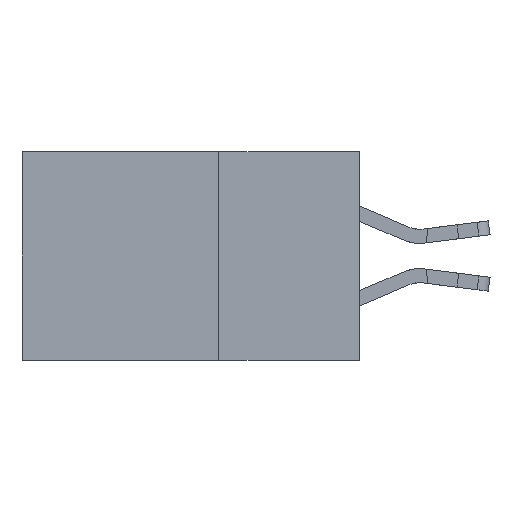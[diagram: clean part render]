
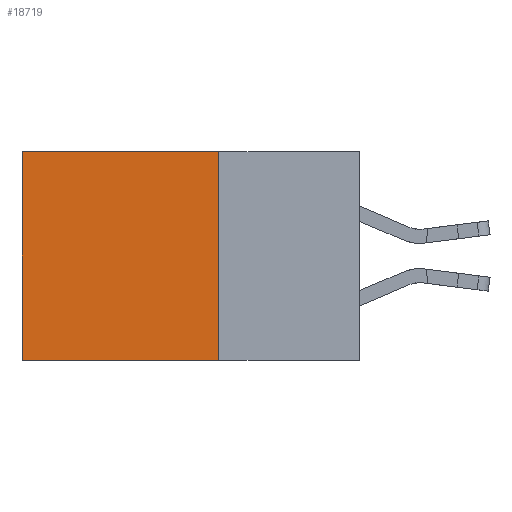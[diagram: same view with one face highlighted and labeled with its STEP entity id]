
A CAD part, left-side view. The second image highlights one B-rep face of the part: STEP entity #18719.
In plain terms, the highlighted planar face has unit normal (-1, 0, 0).
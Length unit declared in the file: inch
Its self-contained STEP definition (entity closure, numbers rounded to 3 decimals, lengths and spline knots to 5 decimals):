
#440 = CARTESIAN_POINT ( 'NONE',  ( 0.2875, 0.25, -0.37 ) ) ;
#581 = DIRECTION ( 'NONE',  ( 0., 1., 0. ) ) ;
#1098 = ORIENTED_EDGE ( 'NONE', *, *, #12425, .T. ) ;
#3612 = CARTESIAN_POINT ( 'NONE',  ( 0.2875, 0.25, -0.37 ) ) ;
#5594 = LINE ( 'NONE', #8821, #17462 ) ;
#5830 = CARTESIAN_POINT ( 'NONE',  ( 0.2875, 0.25, 0. ) ) ;
#5986 = VECTOR ( 'NONE', #22107, 39.37008 ) ;
#6892 = VERTEX_POINT ( 'NONE', #19002 ) ;
#7073 = LINE ( 'NONE', #20081, #5986 ) ;
#7910 = EDGE_CURVE ( 'NONE', #6892, #8746, #5594, .T. ) ;
#8746 = VERTEX_POINT ( 'NONE', #440 ) ;
#8821 = CARTESIAN_POINT ( 'NONE',  ( 0.2875, 0.25, 0. ) ) ;
#9004 = CARTESIAN_POINT ( 'NONE',  ( 0.2875, 0.6, 0. ) ) ;
#9761 = ORIENTED_EDGE ( 'NONE', *, *, #7910, .F. ) ;
#11944 = ORIENTED_EDGE ( 'NONE', *, *, #18707, .F. ) ;
#12171 = VERTEX_POINT ( 'NONE', #9004 ) ;
#12425 = EDGE_CURVE ( 'NONE', #12171, #17841, #19231, .T. ) ;
#13188 = FACE_OUTER_BOUND ( 'NONE', #15187, .T. ) ;
#14242 = DIRECTION ( 'NONE',  ( 0., 0., -1. ) ) ;
#15187 = EDGE_LOOP ( 'NONE', ( #1098, #11944, #9761, #22768 ) ) ;
#15905 = CARTESIAN_POINT ( 'NONE',  ( 0.2875, 0.6, 0. ) ) ;
#17300 = DIRECTION ( 'NONE',  ( 0., 0., -1. ) ) ;
#17462 = VECTOR ( 'NONE', #14242, 39.37008 ) ;
#17841 = VERTEX_POINT ( 'NONE', #19506 ) ;
#17874 = LINE ( 'NONE', #3612, #21955 ) ;
#18110 = DIRECTION ( 'NONE',  ( 0., 0., -1. ) ) ;
#18271 = DIRECTION ( 'NONE',  ( 1., 0., 0. ) ) ;
#18707 = EDGE_CURVE ( 'NONE', #8746, #17841, #17874, .T. ) ;
#18719 = ADVANCED_FACE ( 'NONE', ( #13188 ), #20012, .F. ) ;
#18954 = EDGE_CURVE ( 'NONE', #6892, #12171, #7073, .T. ) ;
#19002 = CARTESIAN_POINT ( 'NONE',  ( 0.2875, 0.25, 0. ) ) ;
#19231 = LINE ( 'NONE', #15905, #19778 ) ;
#19506 = CARTESIAN_POINT ( 'NONE',  ( 0.2875, 0.6, -0.37 ) ) ;
#19778 = VECTOR ( 'NONE', #17300, 39.37008 ) ;
#20012 = PLANE ( 'NONE',  #21965 ) ;
#20081 = CARTESIAN_POINT ( 'NONE',  ( 0.2875, 0.25, 0. ) ) ;
#21955 = VECTOR ( 'NONE', #581, 39.37008 ) ;
#21965 = AXIS2_PLACEMENT_3D ( 'NONE', #5830, #18271, #18110 ) ;
#22107 = DIRECTION ( 'NONE',  ( 0., 1., 0. ) ) ;
#22768 = ORIENTED_EDGE ( 'NONE', *, *, #18954, .T. ) ;
